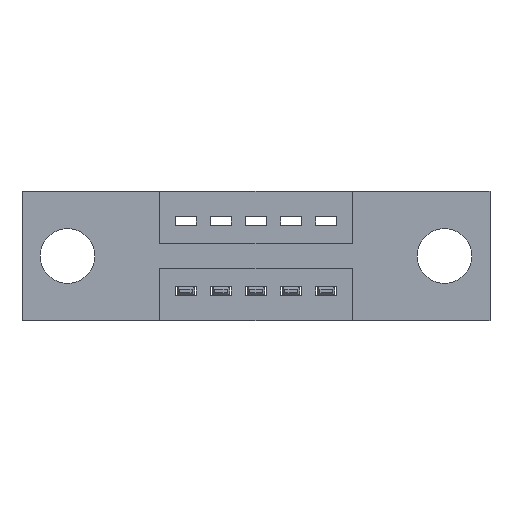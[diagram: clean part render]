
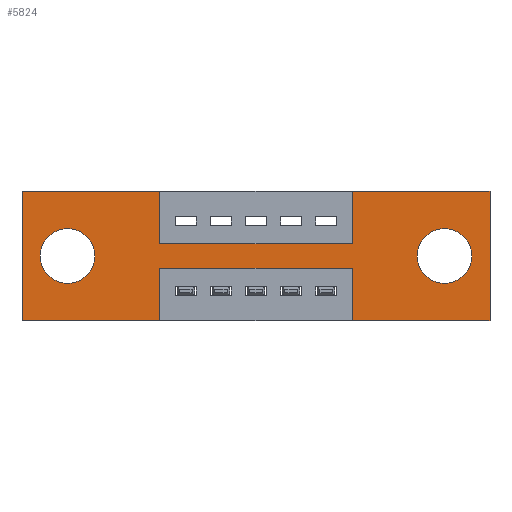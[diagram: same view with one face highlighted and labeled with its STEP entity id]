
A CAD part, front view. The second image highlights one B-rep face of the part: STEP entity #5824.
In plain terms, the highlighted planar face has unit normal (0, -1, 0).
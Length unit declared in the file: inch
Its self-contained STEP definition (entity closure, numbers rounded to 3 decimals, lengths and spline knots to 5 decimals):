
#5 = ORIENTED_EDGE ( 'NONE', *, *, #1173, .F. ) ;
#51 = DIRECTION ( 'NONE',  ( 0., 1., 0. ) ) ;
#82 = LINE ( 'NONE', #980, #5468 ) ;
#107 = LINE ( 'NONE', #6938, #1915 ) ;
#200 = ORIENTED_EDGE ( 'NONE', *, *, #6060, .F. ) ;
#233 = CARTESIAN_POINT ( 'NONE',  ( 0.3925, 0., -0.22 ) ) ;
#255 = CARTESIAN_POINT ( 'NONE',  ( 0.9425, 0., 0. ) ) ;
#275 = VECTOR ( 'NONE', #8306, 39.37008 ) ;
#405 = EDGE_CURVE ( 'NONE', #2091, #4650, #5094, .T. ) ;
#437 = ORIENTED_EDGE ( 'NONE', *, *, #2060, .F. ) ;
#467 = LINE ( 'NONE', #8575, #2480 ) ;
#513 = AXIS2_PLACEMENT_3D ( 'NONE', #8560, #4929, #734 ) ;
#644 = CARTESIAN_POINT ( 'NONE',  ( 0.3925, 0., -0.15 ) ) ;
#733 = DIRECTION ( 'NONE',  ( 0., 0., 1. ) ) ;
#734 = DIRECTION ( 'NONE',  ( 0., 0., -1. ) ) ;
#795 = DIRECTION ( 'NONE',  ( 0., 0., -1. ) ) ;
#822 = EDGE_CURVE ( 'NONE', #6538, #2325, #5893, .T. ) ;
#838 = EDGE_CURVE ( 'NONE', #7146, #5048, #4192, .T. ) ;
#861 = CARTESIAN_POINT ( 'NONE',  ( 0., 0., 0. ) ) ;
#980 = CARTESIAN_POINT ( 'NONE',  ( 0.3925, 0., -0.15 ) ) ;
#984 = VERTEX_POINT ( 'NONE', #2093 ) ;
#1002 = DIRECTION ( 'NONE',  ( 1., 0., 0. ) ) ;
#1050 = ORIENTED_EDGE ( 'NONE', *, *, #838, .F. ) ;
#1056 = CARTESIAN_POINT ( 'NONE',  ( 1.335, 0., 0. ) ) ;
#1152 = VERTEX_POINT ( 'NONE', #3354 ) ;
#1173 = EDGE_CURVE ( 'NONE', #6491, #3346, #8226, .T. ) ;
#1399 = DIRECTION ( 'NONE',  ( 1., 0., 0. ) ) ;
#1496 = CARTESIAN_POINT ( 'NONE',  ( 1.205, 0., -0.107 ) ) ;
#1516 = PLANE ( 'NONE',  #513 ) ;
#1523 = LINE ( 'NONE', #255, #4722 ) ;
#1570 = DIRECTION ( 'NONE',  ( -1., 0., 0. ) ) ;
#1602 = VECTOR ( 'NONE', #6991, 39.37008 ) ;
#1660 = VERTEX_POINT ( 'NONE', #1056 ) ;
#1667 = LINE ( 'NONE', #5822, #6999 ) ;
#1706 = VECTOR ( 'NONE', #5032, 39.37008 ) ;
#1757 = VERTEX_POINT ( 'NONE', #6907 ) ;
#1817 = CARTESIAN_POINT ( 'NONE',  ( 0.9425, 0., -0.37 ) ) ;
#1873 = VERTEX_POINT ( 'NONE', #5069 ) ;
#1915 = VECTOR ( 'NONE', #1399, 39.37008 ) ;
#2049 = DIRECTION ( 'NONE',  ( 0., 1., 0. ) ) ;
#2060 = EDGE_CURVE ( 'NONE', #7786, #6491, #107, .T. ) ;
#2091 = VERTEX_POINT ( 'NONE', #1496 ) ;
#2093 = CARTESIAN_POINT ( 'NONE',  ( 0.13, 0., -0.263 ) ) ;
#2132 = EDGE_CURVE ( 'NONE', #5118, #984, #4884, .T. ) ;
#2209 = CARTESIAN_POINT ( 'NONE',  ( 0.9425, 0., -0.22 ) ) ;
#2257 = CIRCLE ( 'NONE', #7924, 0.078 ) ;
#2325 = VERTEX_POINT ( 'NONE', #1817 ) ;
#2345 = AXIS2_PLACEMENT_3D ( 'NONE', #7596, #7779, #795 ) ;
#2480 = VECTOR ( 'NONE', #4272, 39.37008 ) ;
#2497 = DIRECTION ( 'NONE',  ( -1., 0., 0. ) ) ;
#2674 = DIRECTION ( 'NONE',  ( 0., 0., 1. ) ) ;
#2704 = DIRECTION ( 'NONE',  ( 0., 1., 0. ) ) ;
#2713 = EDGE_CURVE ( 'NONE', #984, #5118, #2257, .T. ) ;
#2729 = CARTESIAN_POINT ( 'NONE',  ( 0.13, 0., -0.185 ) ) ;
#2795 = ORIENTED_EDGE ( 'NONE', *, *, #8242, .F. ) ;
#3173 = LINE ( 'NONE', #7099, #6423 ) ;
#3320 = EDGE_CURVE ( 'NONE', #3346, #1152, #82, .T. ) ;
#3346 = VERTEX_POINT ( 'NONE', #644 ) ;
#3354 = CARTESIAN_POINT ( 'NONE',  ( 0.9425, 0., -0.15 ) ) ;
#3391 = ORIENTED_EDGE ( 'NONE', *, *, #4060, .F. ) ;
#3442 = CARTESIAN_POINT ( 'NONE',  ( 0.13, 0., -0.185 ) ) ;
#3461 = FACE_OUTER_BOUND ( 'NONE', #8374, .T. ) ;
#3537 = LINE ( 'NONE', #8084, #5079 ) ;
#3547 = ORIENTED_EDGE ( 'NONE', *, *, #7706, .F. ) ;
#3983 = LINE ( 'NONE', #861, #1706 ) ;
#4041 = CARTESIAN_POINT ( 'NONE',  ( 0., 0., -0.37 ) ) ;
#4060 = EDGE_CURVE ( 'NONE', #1660, #6538, #1667, .T. ) ;
#4134 = EDGE_CURVE ( 'NONE', #5048, #1873, #3173, .T. ) ;
#4174 = CARTESIAN_POINT ( 'NONE',  ( 0.9425, 0., 0. ) ) ;
#4192 = LINE ( 'NONE', #233, #7316 ) ;
#4272 = DIRECTION ( 'NONE',  ( 0., 0., 1. ) ) ;
#4650 = VERTEX_POINT ( 'NONE', #6341 ) ;
#4670 = CARTESIAN_POINT ( 'NONE',  ( 0.9425, 0., -0.37 ) ) ;
#4722 = VECTOR ( 'NONE', #7626, 39.37008 ) ;
#4766 = ORIENTED_EDGE ( 'NONE', *, *, #6203, .F. ) ;
#4880 = CARTESIAN_POINT ( 'NONE',  ( 0.13, 0., -0.107 ) ) ;
#4884 = CIRCLE ( 'NONE', #7412, 0.078 ) ;
#4889 = CARTESIAN_POINT ( 'NONE',  ( 0.3925, 0., 0. ) ) ;
#4929 = DIRECTION ( 'NONE',  ( 0., -1., 0. ) ) ;
#5032 = DIRECTION ( 'NONE',  ( 1., 0., 0. ) ) ;
#5048 = VERTEX_POINT ( 'NONE', #6690 ) ;
#5069 = CARTESIAN_POINT ( 'NONE',  ( 0.3925, 0., -0.37 ) ) ;
#5079 = VECTOR ( 'NONE', #6303, 39.37008 ) ;
#5094 = CIRCLE ( 'NONE', #2345, 0.078 ) ;
#5118 = VERTEX_POINT ( 'NONE', #4880 ) ;
#5146 = DIRECTION ( 'NONE',  ( 0., 0., -1. ) ) ;
#5230 = FACE_BOUND ( 'NONE', #8446, .T. ) ;
#5262 = DIRECTION ( 'NONE',  ( 0., 0., -1. ) ) ;
#5359 = ORIENTED_EDGE ( 'NONE', *, *, #7017, .T. ) ;
#5424 = LINE ( 'NONE', #4670, #275 ) ;
#5467 = ORIENTED_EDGE ( 'NONE', *, *, #4134, .F. ) ;
#5468 = VECTOR ( 'NONE', #1002, 39.37008 ) ;
#5563 = EDGE_LOOP ( 'NONE', ( #8561, #8110 ) ) ;
#5762 = CARTESIAN_POINT ( 'NONE',  ( 0., 0., 0. ) ) ;
#5766 = ORIENTED_EDGE ( 'NONE', *, *, #3320, .F. ) ;
#5805 = CIRCLE ( 'NONE', #8548, 0.078 ) ;
#5822 = CARTESIAN_POINT ( 'NONE',  ( 1.335, 0., 0. ) ) ;
#5824 = ADVANCED_FACE ( 'NONE', ( #5230, #6883, #3461 ), #1516, .T. ) ;
#5893 = LINE ( 'NONE', #4041, #7490 ) ;
#6017 = CARTESIAN_POINT ( 'NONE',  ( 1.205, 0., -0.185 ) ) ;
#6060 = EDGE_CURVE ( 'NONE', #1152, #7100, #1523, .T. ) ;
#6203 = EDGE_CURVE ( 'NONE', #2325, #7146, #5424, .T. ) ;
#6303 = DIRECTION ( 'NONE',  ( -1., 0., 0. ) ) ;
#6341 = CARTESIAN_POINT ( 'NONE',  ( 1.205, 0., -0.263 ) ) ;
#6423 = VECTOR ( 'NONE', #5262, 39.37008 ) ;
#6427 = ORIENTED_EDGE ( 'NONE', *, *, #405, .T. ) ;
#6491 = VERTEX_POINT ( 'NONE', #4889 ) ;
#6538 = VERTEX_POINT ( 'NONE', #7997 ) ;
#6634 = DIRECTION ( 'NONE',  ( 0., 0., -1. ) ) ;
#6690 = CARTESIAN_POINT ( 'NONE',  ( 0.3925, 0., -0.22 ) ) ;
#6819 = ORIENTED_EDGE ( 'NONE', *, *, #7698, .F. ) ;
#6883 = FACE_BOUND ( 'NONE', #5563, .T. ) ;
#6907 = CARTESIAN_POINT ( 'NONE',  ( 0., 0., -0.37 ) ) ;
#6938 = CARTESIAN_POINT ( 'NONE',  ( 0., 0., 0. ) ) ;
#6991 = DIRECTION ( 'NONE',  ( 0., 0., -1. ) ) ;
#6999 = VECTOR ( 'NONE', #5146, 39.37008 ) ;
#7017 = EDGE_CURVE ( 'NONE', #4650, #2091, #5805, .T. ) ;
#7026 = CARTESIAN_POINT ( 'NONE',  ( 0.3925, 0., 0. ) ) ;
#7099 = CARTESIAN_POINT ( 'NONE',  ( 0.3925, 0., -0.37 ) ) ;
#7100 = VERTEX_POINT ( 'NONE', #4174 ) ;
#7146 = VERTEX_POINT ( 'NONE', #2209 ) ;
#7316 = VECTOR ( 'NONE', #2497, 39.37008 ) ;
#7412 = AXIS2_PLACEMENT_3D ( 'NONE', #3442, #51, #733 ) ;
#7490 = VECTOR ( 'NONE', #1570, 39.37008 ) ;
#7596 = CARTESIAN_POINT ( 'NONE',  ( 1.205, 0., -0.185 ) ) ;
#7626 = DIRECTION ( 'NONE',  ( 0., 0., 1. ) ) ;
#7698 = EDGE_CURVE ( 'NONE', #7100, #1660, #3983, .T. ) ;
#7706 = EDGE_CURVE ( 'NONE', #1873, #1757, #3537, .T. ) ;
#7779 = DIRECTION ( 'NONE',  ( 0., 1., 0. ) ) ;
#7786 = VERTEX_POINT ( 'NONE', #5762 ) ;
#7924 = AXIS2_PLACEMENT_3D ( 'NONE', #2729, #2704, #2674 ) ;
#7997 = CARTESIAN_POINT ( 'NONE',  ( 1.335, 0., -0.37 ) ) ;
#8084 = CARTESIAN_POINT ( 'NONE',  ( 0., 0., -0.37 ) ) ;
#8110 = ORIENTED_EDGE ( 'NONE', *, *, #2713, .T. ) ;
#8207 = ORIENTED_EDGE ( 'NONE', *, *, #822, .F. ) ;
#8226 = LINE ( 'NONE', #7026, #1602 ) ;
#8242 = EDGE_CURVE ( 'NONE', #1757, #7786, #467, .T. ) ;
#8306 = DIRECTION ( 'NONE',  ( 0., 0., 1. ) ) ;
#8374 = EDGE_LOOP ( 'NONE', ( #5467, #1050, #4766, #8207, #3391, #6819, #200, #5766, #5, #437, #2795, #3547 ) ) ;
#8446 = EDGE_LOOP ( 'NONE', ( #6427, #5359 ) ) ;
#8548 = AXIS2_PLACEMENT_3D ( 'NONE', #6017, #2049, #6634 ) ;
#8560 = CARTESIAN_POINT ( 'NONE',  ( 0., 0., -0.37 ) ) ;
#8561 = ORIENTED_EDGE ( 'NONE', *, *, #2132, .T. ) ;
#8575 = CARTESIAN_POINT ( 'NONE',  ( 0., 0., 0. ) ) ;
